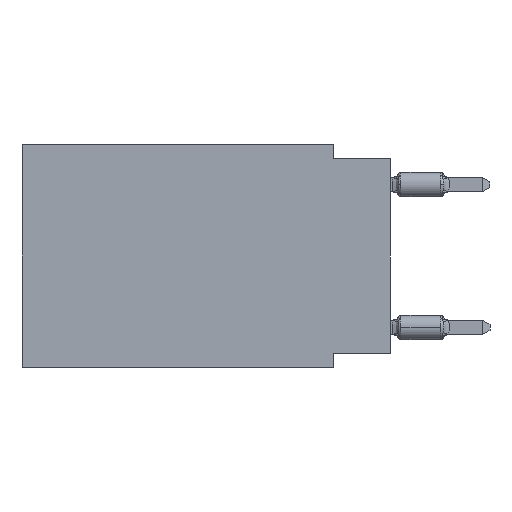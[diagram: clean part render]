
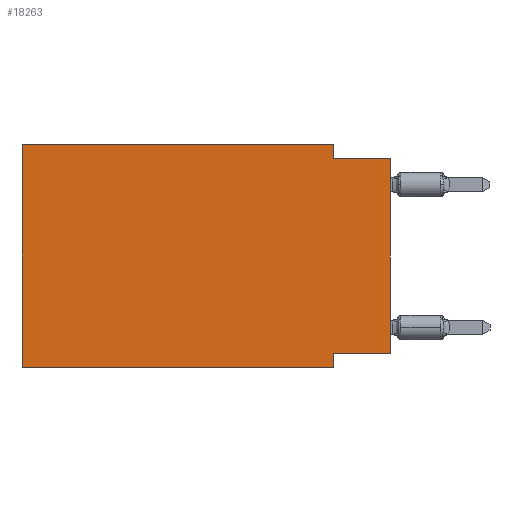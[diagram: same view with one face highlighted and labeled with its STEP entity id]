
A CAD part, left-side view. The second image highlights one B-rep face of the part: STEP entity #18263.
In plain terms, the highlighted planar face has unit normal (-1, 0, 0).
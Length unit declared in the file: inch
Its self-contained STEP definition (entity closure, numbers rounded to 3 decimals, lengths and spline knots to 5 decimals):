
#2104 = EDGE_LOOP ( 'NONE', ( #28770, #9619, #25906, #39770, #24442, #17773, #36726, #3938 ) ) ;
#2174 = EDGE_CURVE ( 'NONE', #28949, #24345, #37128, .T. ) ;
#2358 = VECTOR ( 'NONE', #29111, 39.37008 ) ;
#2392 = DIRECTION ( 'NONE',  ( 0., -1., 0. ) ) ;
#2952 = EDGE_CURVE ( 'NONE', #38625, #33930, #39566, .T. ) ;
#3001 = LINE ( 'NONE', #28012, #21331 ) ;
#3938 = ORIENTED_EDGE ( 'NONE', *, *, #16319, .F. ) ;
#4121 = VECTOR ( 'NONE', #27325, 39.37008 ) ;
#6612 = VERTEX_POINT ( 'NONE', #33997 ) ;
#7155 = LINE ( 'NONE', #32588, #8342 ) ;
#8342 = VECTOR ( 'NONE', #35472, 39.37008 ) ;
#9619 = ORIENTED_EDGE ( 'NONE', *, *, #36328, .F. ) ;
#11452 = FACE_OUTER_BOUND ( 'NONE', #2104, .T. ) ;
#11652 = DIRECTION ( 'NONE',  ( 0., 0., -1. ) ) ;
#12223 = EDGE_CURVE ( 'NONE', #6612, #34693, #22652, .T. ) ;
#12288 = DIRECTION ( 'NONE',  ( 0., 0., 1. ) ) ;
#14829 = CARTESIAN_POINT ( 'NONE',  ( 0., 0.645, -0.39 ) ) ;
#14868 = EDGE_CURVE ( 'NONE', #35200, #24345, #7155, .T. ) ;
#14981 = CARTESIAN_POINT ( 'NONE',  ( 0., 0.645, 0. ) ) ;
#16319 = EDGE_CURVE ( 'NONE', #6612, #35200, #28149, .T. ) ;
#16324 = CARTESIAN_POINT ( 'NONE',  ( 0., 0.1, 0. ) ) ;
#17773 = ORIENTED_EDGE ( 'NONE', *, *, #2174, .T. ) ;
#18141 = LINE ( 'NONE', #40441, #32037 ) ;
#18263 = ADVANCED_FACE ( 'NONE', ( #11452 ), #22745, .F. ) ;
#19627 = DIRECTION ( 'NONE',  ( 1., 0., 0. ) ) ;
#20613 = CARTESIAN_POINT ( 'NONE',  ( 0., 0.645, 0. ) ) ;
#21331 = VECTOR ( 'NONE', #2392, 39.37008 ) ;
#22652 = LINE ( 'NONE', #32852, #2358 ) ;
#22745 = PLANE ( 'NONE',  #24503 ) ;
#24345 = VERTEX_POINT ( 'NONE', #36469 ) ;
#24442 = ORIENTED_EDGE ( 'NONE', *, *, #37279, .F. ) ;
#24503 = AXIS2_PLACEMENT_3D ( 'NONE', #35451, #19627, #11652 ) ;
#25744 = VECTOR ( 'NONE', #31956, 39.37008 ) ;
#25906 = ORIENTED_EDGE ( 'NONE', *, *, #31989, .F. ) ;
#26098 = VERTEX_POINT ( 'NONE', #31484 ) ;
#27325 = DIRECTION ( 'NONE',  ( 0., -1., 0. ) ) ;
#27710 = CARTESIAN_POINT ( 'NONE',  ( 0., 0.1, 0. ) ) ;
#28012 = CARTESIAN_POINT ( 'NONE',  ( 0., 0., -0.025 ) ) ;
#28149 = LINE ( 'NONE', #28772, #31726 ) ;
#28770 = ORIENTED_EDGE ( 'NONE', *, *, #12223, .T. ) ;
#28772 = CARTESIAN_POINT ( 'NONE',  ( 0., 0., -0.365 ) ) ;
#28804 = VECTOR ( 'NONE', #36856, 39.37008 ) ;
#28949 = VERTEX_POINT ( 'NONE', #31657 ) ;
#29111 = DIRECTION ( 'NONE',  ( 0., 0., 1. ) ) ;
#31484 = CARTESIAN_POINT ( 'NONE',  ( 0., 0.1, -0.025 ) ) ;
#31657 = CARTESIAN_POINT ( 'NONE',  ( 0., 0.645, -0.39 ) ) ;
#31726 = VECTOR ( 'NONE', #37969, 39.37008 ) ;
#31956 = DIRECTION ( 'NONE',  ( 0., 0., -1. ) ) ;
#31989 = EDGE_CURVE ( 'NONE', #33930, #26098, #32365, .T. ) ;
#32037 = VECTOR ( 'NONE', #12288, 39.37008 ) ;
#32365 = LINE ( 'NONE', #16324, #25744 ) ;
#32588 = CARTESIAN_POINT ( 'NONE',  ( 0., 0.1, -0.39 ) ) ;
#32852 = CARTESIAN_POINT ( 'NONE',  ( 0., 0., 0. ) ) ;
#33930 = VERTEX_POINT ( 'NONE', #27710 ) ;
#33997 = CARTESIAN_POINT ( 'NONE',  ( 0., 0., -0.365 ) ) ;
#34693 = VERTEX_POINT ( 'NONE', #37248 ) ;
#35200 = VERTEX_POINT ( 'NONE', #41135 ) ;
#35451 = CARTESIAN_POINT ( 'NONE',  ( 0., 0.645, 0. ) ) ;
#35472 = DIRECTION ( 'NONE',  ( 0., 0., -1. ) ) ;
#36328 = EDGE_CURVE ( 'NONE', #26098, #34693, #3001, .T. ) ;
#36469 = CARTESIAN_POINT ( 'NONE',  ( 0., 0.1, -0.39 ) ) ;
#36726 = ORIENTED_EDGE ( 'NONE', *, *, #14868, .F. ) ;
#36856 = DIRECTION ( 'NONE',  ( 0., -1., 0. ) ) ;
#37128 = LINE ( 'NONE', #14829, #4121 ) ;
#37248 = CARTESIAN_POINT ( 'NONE',  ( 0., 0., -0.025 ) ) ;
#37279 = EDGE_CURVE ( 'NONE', #28949, #38625, #18141, .T. ) ;
#37969 = DIRECTION ( 'NONE',  ( 0., 1., 0. ) ) ;
#38625 = VERTEX_POINT ( 'NONE', #14981 ) ;
#39566 = LINE ( 'NONE', #20613, #28804 ) ;
#39770 = ORIENTED_EDGE ( 'NONE', *, *, #2952, .F. ) ;
#40441 = CARTESIAN_POINT ( 'NONE',  ( 0., 0.645, 0. ) ) ;
#41135 = CARTESIAN_POINT ( 'NONE',  ( 0., 0.1, -0.365 ) ) ;
